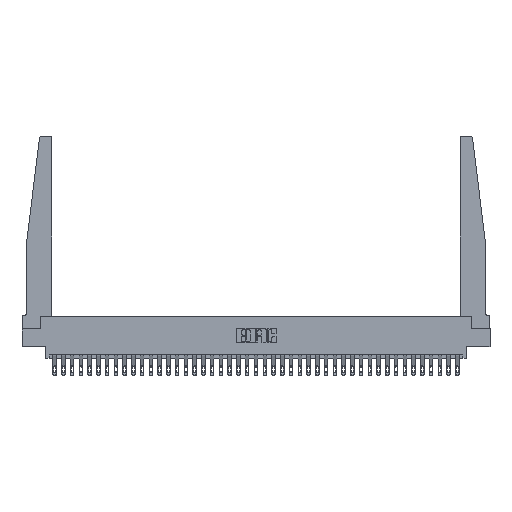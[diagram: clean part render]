
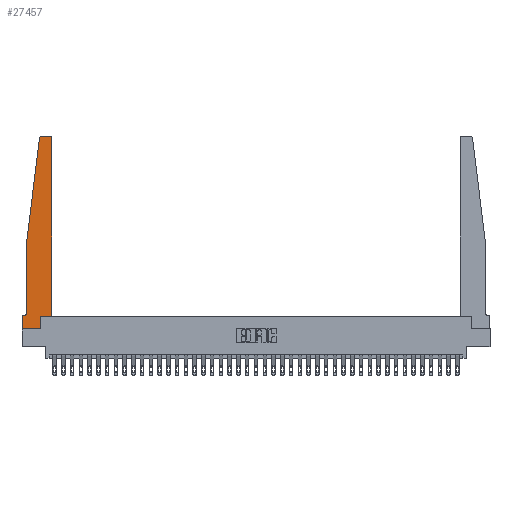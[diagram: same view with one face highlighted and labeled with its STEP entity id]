
A CAD part, top view. The second image highlights one B-rep face of the part: STEP entity #27457.
In plain terms, the highlighted planar face has unit normal (0, 0, 1).
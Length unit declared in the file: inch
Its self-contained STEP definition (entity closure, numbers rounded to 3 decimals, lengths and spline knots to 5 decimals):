
#154 = ORIENTED_EDGE ( 'NONE', *, *, #35236, .T. ) ;
#219 = FACE_OUTER_BOUND ( 'NONE', #1292, .T. ) ;
#453 = AXIS2_PLACEMENT_3D ( 'NONE', #8433, #27398, #11166 ) ;
#619 = CARTESIAN_POINT ( 'NONE',  ( 0.065, 1.25, 0.37 ) ) ;
#1067 = EDGE_CURVE ( 'NONE', #18032, #18191, #22247, .T. ) ;
#1292 = EDGE_LOOP ( 'NONE', ( #9573, #2441, #9826, #33564, #21845, #30499, #154, #12365, #8034, #22238, #7715, #27805 ) ) ;
#1691 = CARTESIAN_POINT ( 'NONE',  ( 0.065, 0.1875, 0.37 ) ) ;
#1886 = CARTESIAN_POINT ( 'NONE',  ( 0.2605, 0.18, 0.37 ) ) ;
#2339 = DIRECTION ( 'NONE',  ( -0.122, -0.992, 0. ) ) ;
#2441 = ORIENTED_EDGE ( 'NONE', *, *, #31461, .T. ) ;
#2879 = VERTEX_POINT ( 'NONE', #15207 ) ;
#3642 = CARTESIAN_POINT ( 'NONE',  ( 0.425, 0.18, 0.37 ) ) ;
#3921 = DIRECTION ( 'NONE',  ( 0., 0., 1. ) ) ;
#5245 = LINE ( 'NONE', #9700, #18852 ) ;
#5507 = EDGE_CURVE ( 'NONE', #34187, #30552, #33526, .T. ) ;
#6328 = LINE ( 'NONE', #7693, #34439 ) ;
#6942 = DIRECTION ( 'NONE',  ( 0., -1., 0. ) ) ;
#7026 = PLANE ( 'NONE',  #20149 ) ;
#7075 = EDGE_CURVE ( 'NONE', #18191, #17577, #26999, .T. ) ;
#7180 = DIRECTION ( 'NONE',  ( -1., 0., 0. ) ) ;
#7693 = CARTESIAN_POINT ( 'NONE',  ( 0.425, 0.18, 0.37 ) ) ;
#7715 = ORIENTED_EDGE ( 'NONE', *, *, #30166, .T. ) ;
#8034 = ORIENTED_EDGE ( 'NONE', *, *, #8879, .T. ) ;
#8117 = CARTESIAN_POINT ( 'NONE',  ( 0.25, 2.75, 0.37 ) ) ;
#8433 = CARTESIAN_POINT ( 'NONE',  ( 0.395, 2.72, 0.37 ) ) ;
#8879 = EDGE_CURVE ( 'NONE', #30552, #33016, #23057, .T. ) ;
#9573 = ORIENTED_EDGE ( 'NONE', *, *, #19116, .T. ) ;
#9700 = CARTESIAN_POINT ( 'NONE',  ( 0., 0., 0.37 ) ) ;
#9826 = ORIENTED_EDGE ( 'NONE', *, *, #23153, .T. ) ;
#10604 = VECTOR ( 'NONE', #10862, 39.37008 ) ;
#10669 = CIRCLE ( 'NONE', #27247, 0.03 ) ;
#10862 = DIRECTION ( 'NONE',  ( -1., 0., 0. ) ) ;
#11166 = DIRECTION ( 'NONE',  ( 1., 0., 0. ) ) ;
#12365 = ORIENTED_EDGE ( 'NONE', *, *, #5507, .T. ) ;
#12514 = DIRECTION ( 'NONE',  ( 0., 0., 1. ) ) ;
#13521 = VERTEX_POINT ( 'NONE', #19750 ) ;
#13983 = CARTESIAN_POINT ( 'NONE',  ( 0.015, 0.2375, 0.37 ) ) ;
#14217 = VERTEX_POINT ( 'NONE', #25070 ) ;
#14226 = DIRECTION ( 'NONE',  ( 0., -1., 0. ) ) ;
#15207 = CARTESIAN_POINT ( 'NONE',  ( 0., 0.1875, 0.37 ) ) ;
#15341 = DIRECTION ( 'NONE',  ( 0., 1., 0. ) ) ;
#15923 = CARTESIAN_POINT ( 'NONE',  ( 0.065, 1.25, 0.37 ) ) ;
#16683 = DIRECTION ( 'NONE',  ( -1., 0., 0. ) ) ;
#16687 = VECTOR ( 'NONE', #15341, 39.37008 ) ;
#17577 = VERTEX_POINT ( 'NONE', #25187 ) ;
#17847 = DIRECTION ( 'NONE',  ( 1., 0., 0. ) ) ;
#18032 = VERTEX_POINT ( 'NONE', #29714 ) ;
#18191 = VERTEX_POINT ( 'NONE', #30183 ) ;
#18852 = VECTOR ( 'NONE', #6942, 39.37008 ) ;
#19116 = EDGE_CURVE ( 'NONE', #27264, #28963, #32290, .T. ) ;
#19750 = CARTESIAN_POINT ( 'NONE',  ( 0.24675, 2.72367, 0.37 ) ) ;
#20077 = VECTOR ( 'NONE', #2339, 39.37008 ) ;
#20149 = AXIS2_PLACEMENT_3D ( 'NONE', #28771, #12514, #31530 ) ;
#20227 = CARTESIAN_POINT ( 'NONE',  ( 0.27653, 2.72, 0.37 ) ) ;
#20560 = LINE ( 'NONE', #1691, #34202 ) ;
#21412 = VECTOR ( 'NONE', #14226, 39.37008 ) ;
#21845 = ORIENTED_EDGE ( 'NONE', *, *, #7075, .T. ) ;
#22238 = ORIENTED_EDGE ( 'NONE', *, *, #25019, .T. ) ;
#22247 = LINE ( 'NONE', #619, #21412 ) ;
#22325 = EDGE_CURVE ( 'NONE', #31655, #27264, #32091, .T. ) ;
#22697 = CARTESIAN_POINT ( 'NONE',  ( 0.395, 2.75, 0.37 ) ) ;
#22930 = DIRECTION ( 'NONE',  ( 1., 0., 0. ) ) ;
#23057 = LINE ( 'NONE', #1886, #16687 ) ;
#23153 = EDGE_CURVE ( 'NONE', #13521, #18032, #27280, .T. ) ;
#25019 = EDGE_CURVE ( 'NONE', #33016, #14217, #6328, .T. ) ;
#25070 = CARTESIAN_POINT ( 'NONE',  ( 0.425, 0.18, 0.37 ) ) ;
#25187 = CARTESIAN_POINT ( 'NONE',  ( 0.015, 0.1875, 0.37 ) ) ;
#25371 = DIRECTION ( 'NONE',  ( 0., 1., 0. ) ) ;
#25944 = VECTOR ( 'NONE', #25371, 39.37008 ) ;
#26999 = CIRCLE ( 'NONE', #33300, 0.05 ) ;
#27084 = VECTOR ( 'NONE', #17847, 39.37008 ) ;
#27146 = CARTESIAN_POINT ( 'NONE',  ( 0., 0., 0.37 ) ) ;
#27247 = AXIS2_PLACEMENT_3D ( 'NONE', #20227, #3921, #22930 ) ;
#27264 = VERTEX_POINT ( 'NONE', #22697 ) ;
#27280 = LINE ( 'NONE', #15923, #20077 ) ;
#27398 = DIRECTION ( 'NONE',  ( 0., 0., 1. ) ) ;
#27457 = ADVANCED_FACE ( 'NONE', ( #219 ), #7026, .T. ) ;
#27805 = ORIENTED_EDGE ( 'NONE', *, *, #22325, .T. ) ;
#27836 = CARTESIAN_POINT ( 'NONE',  ( 0.2605, 0.18, 0.37 ) ) ;
#28329 = CARTESIAN_POINT ( 'NONE',  ( 0.27653, 2.75, 0.37 ) ) ;
#28691 = EDGE_CURVE ( 'NONE', #17577, #2879, #20560, .T. ) ;
#28771 = CARTESIAN_POINT ( 'NONE',  ( 0., 0.1875, 0.37 ) ) ;
#28963 = VERTEX_POINT ( 'NONE', #28329 ) ;
#29564 = CARTESIAN_POINT ( 'NONE',  ( 0.2605, 0., 0.37 ) ) ;
#29714 = CARTESIAN_POINT ( 'NONE',  ( 0.065, 1.25, 0.37 ) ) ;
#30166 = EDGE_CURVE ( 'NONE', #14217, #31655, #32396, .T. ) ;
#30183 = CARTESIAN_POINT ( 'NONE',  ( 0.065, 0.2375, 0.37 ) ) ;
#30499 = ORIENTED_EDGE ( 'NONE', *, *, #28691, .T. ) ;
#30552 = VERTEX_POINT ( 'NONE', #29564 ) ;
#31461 = EDGE_CURVE ( 'NONE', #28963, #13521, #10669, .T. ) ;
#31530 = DIRECTION ( 'NONE',  ( 1., 0., 0. ) ) ;
#31648 = CARTESIAN_POINT ( 'NONE',  ( 0.425, 2.72, 0.37 ) ) ;
#31655 = VERTEX_POINT ( 'NONE', #31648 ) ;
#32088 = DIRECTION ( 'NONE',  ( 1., 0., 0. ) ) ;
#32091 = CIRCLE ( 'NONE', #453, 0.03 ) ;
#32290 = LINE ( 'NONE', #8117, #10604 ) ;
#32396 = LINE ( 'NONE', #3642, #25944 ) ;
#33006 = DIRECTION ( 'NONE',  ( 0., 0., -1. ) ) ;
#33016 = VERTEX_POINT ( 'NONE', #27836 ) ;
#33300 = AXIS2_PLACEMENT_3D ( 'NONE', #13983, #33006, #16683 ) ;
#33526 = LINE ( 'NONE', #34157, #27084 ) ;
#33564 = ORIENTED_EDGE ( 'NONE', *, *, #1067, .T. ) ;
#34157 = CARTESIAN_POINT ( 'NONE',  ( 0., 0., 0.37 ) ) ;
#34187 = VERTEX_POINT ( 'NONE', #27146 ) ;
#34202 = VECTOR ( 'NONE', #7180, 39.37008 ) ;
#34439 = VECTOR ( 'NONE', #32088, 39.37008 ) ;
#35236 = EDGE_CURVE ( 'NONE', #2879, #34187, #5245, .T. ) ;
